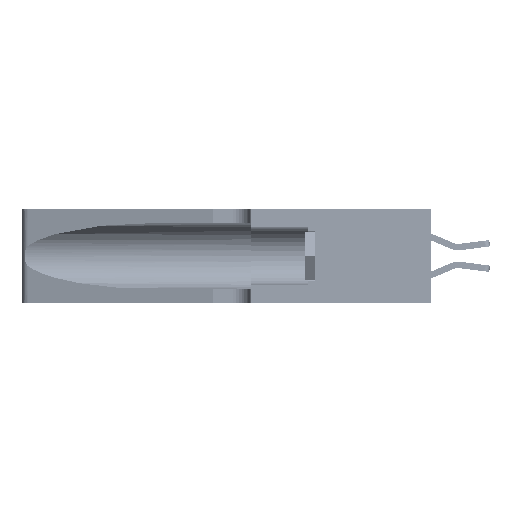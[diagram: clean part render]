
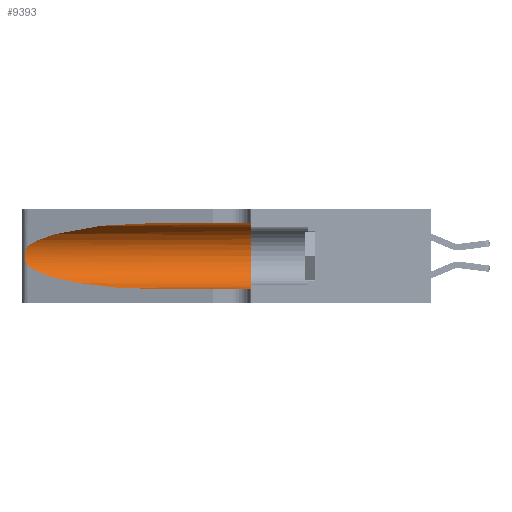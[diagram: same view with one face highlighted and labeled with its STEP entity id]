
A CAD part, left-side view. The second image highlights one B-rep face of the part: STEP entity #9393.
In plain terms, the highlighted cylindrical face has radius 3.308 mm (diameter 6.617 mm), a partial arc.
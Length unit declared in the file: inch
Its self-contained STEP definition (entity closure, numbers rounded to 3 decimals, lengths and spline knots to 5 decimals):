
#1543 = DIRECTION ( 'NONE',  ( 0., 0., 1. ) ) ;
#2768 = AXIS2_PLACEMENT_3D ( 'NONE', #37873, #28418, #1543 ) ;
#3234 = VECTOR ( 'NONE', #26220, 39.37008 ) ;
#3372 = CARTESIAN_POINT ( 'NONE',  ( 0.26017, 1.23833, 0.17102 ) ) ;
#3890 = CARTESIAN_POINT ( 'NONE',  ( 0.25787, 1.23484, 0.2124 ) ) ;
#4260 = VERTEX_POINT ( 'NONE', #5077 ) ;
#5077 = CARTESIAN_POINT ( 'NONE',  ( 0.25487, 1.22718, 0.14631 ) ) ;
#5618 = EDGE_CURVE ( 'NONE', #32539, #18582, #40842, .T. ) ;
#5830 = DIRECTION ( 'NONE',  ( 0., -1., 0. ) ) ;
#6463 = ORIENTED_EDGE ( 'NONE', *, *, #34901, .T. ) ;
#6616 = CARTESIAN_POINT ( 'NONE',  ( 0.18966, 0.96281, 0.31525 ) ) ;
#7053 = ORIENTED_EDGE ( 'NONE', *, *, #42344, .F. ) ;
#7362 = ORIENTED_EDGE ( 'NONE', *, *, #5618, .F. ) ;
#7953 = CARTESIAN_POINT ( 'NONE',  ( 0.25639, 1.23186, 0.15144 ) ) ;
#8888 = CARTESIAN_POINT ( 'NONE',  ( 0.1305, 0.35, 0.31525 ) ) ;
#9348 = CARTESIAN_POINT ( 'NONE',  ( 0.1305, 0.72297, 0.31525 ) ) ;
#9393 = ADVANCED_FACE ( 'NONE', ( #14552 ), #27789, .F. ) ;
#9564 = DIRECTION ( 'NONE',  ( 0., 0., -1. ) ) ;
#11180 = EDGE_CURVE ( 'NONE', #30647, #4260, #34454, .T. ) ;
#14552 = FACE_OUTER_BOUND ( 'NONE', #50273, .T. ) ;
#14632 = CARTESIAN_POINT ( 'NONE',  ( 0.1305, 0.72297, 0.31525 ) ) ;
#15154 = CARTESIAN_POINT ( 'NONE',  ( 0.25487, 1.22718, 0.22369 ) ) ;
#15461 = CARTESIAN_POINT ( 'NONE',  ( 0.25487, 1.22718, 0.22369 ) ) ;
#15671 = DIRECTION ( 'NONE',  ( 0., -1., 0. ) ) ;
#15989 = CARTESIAN_POINT ( 'NONE',  ( 0.26075, 1.23896, 0.19203 ) ) ;
#16619 = CARTESIAN_POINT ( 'NONE',  ( 0.25487, 1.22718, 0.14631 ) ) ;
#17465 = ORIENTED_EDGE ( 'NONE', *, *, #11180, .T. ) ;
#17618 = CARTESIAN_POINT ( 'NONE',  ( 0.1305, 1.61858, 0.05475 ) ) ;
#18582 = VERTEX_POINT ( 'NONE', #36812 ) ;
#19535 = AXIS2_PLACEMENT_3D ( 'NONE', #50505, #5830, #9564 ) ;
#25930 =( BOUNDED_CURVE ( )  B_SPLINE_CURVE ( 3, ( #14632, #6616, #43300, #15154 ),
 .UNSPECIFIED., .F., .F. ) 
 B_SPLINE_CURVE_WITH_KNOTS ( ( 4, 4 ),
 ( 1.5708, 2.84003 ),
 .UNSPECIFIED. ) 
 CURVE ( )  GEOMETRIC_REPRESENTATION_ITEM ( )  RATIONAL_B_SPLINE_CURVE ( ( 1., 0.87, 0.87, 1. ) ) 
 REPRESENTATION_ITEM ( '' )  );
#26193 = VERTEX_POINT ( 'NONE', #9348 ) ;
#26220 = DIRECTION ( 'NONE',  ( 0., -1., 0. ) ) ;
#27789 = CYLINDRICAL_SURFACE ( 'NONE', #19535, 0.13025 ) ;
#27816 = CARTESIAN_POINT ( 'NONE',  ( 0.25856, 1.23593, 0.16098 ) ) ;
#28418 = DIRECTION ( 'NONE',  ( 0., 1., 0. ) ) ;
#29225 = LINE ( 'NONE', #17618, #3234 ) ;
#30647 = VERTEX_POINT ( 'NONE', #37990 ) ;
#30667 = EDGE_CURVE ( 'NONE', #36294, #18582, #29225, .T. ) ;
#31730 = CARTESIAN_POINT ( 'NONE',  ( 0.25789, 1.23486, 0.15765 ) ) ;
#32107 =( BOUNDED_CURVE ( )  B_SPLINE_CURVE ( 3, ( #16619, #44578, #41038, #45284 ),
 .UNSPECIFIED., .F., .F. ) 
 B_SPLINE_CURVE_WITH_KNOTS ( ( 4, 4 ),
 ( 3.44316, 4.71239 ),
 .UNSPECIFIED. ) 
 CURVE ( )  GEOMETRIC_REPRESENTATION_ITEM ( )  RATIONAL_B_SPLINE_CURVE ( ( 1., 0.87, 0.87, 1. ) ) 
 REPRESENTATION_ITEM ( '' )  );
#32539 = VERTEX_POINT ( 'NONE', #8888 ) ;
#34454 = B_SPLINE_CURVE_WITH_KNOTS ( 'NONE', 3,
 ( #15461, #43767, #36178, #3890, #47700, #51940, #15989, #39579, #3372, #27816, #31730, #7953, #35656, #44119 ),
 .UNSPECIFIED., .F., .F.,
 ( 4, 2, 2, 2, 2, 2, 4 ),
 ( 0., 0.00027, 0.00053, 0.00107, 0.0016, 0.00187, 0.00214 ),
 .UNSPECIFIED. ) ;
#34901 = EDGE_CURVE ( 'NONE', #26193, #30647, #25930, .T. ) ;
#35656 = CARTESIAN_POINT ( 'NONE',  ( 0.25555, 1.22993, 0.14849 ) ) ;
#36178 = CARTESIAN_POINT ( 'NONE',  ( 0.25639, 1.23184, 0.21858 ) ) ;
#36294 = VERTEX_POINT ( 'NONE', #40643 ) ;
#36812 = CARTESIAN_POINT ( 'NONE',  ( 0.1305, 0.35, 0.05475 ) ) ;
#37873 = CARTESIAN_POINT ( 'NONE',  ( 0.1305, 0.35, 0.185 ) ) ;
#37990 = CARTESIAN_POINT ( 'NONE',  ( 0.25487, 1.22718, 0.22369 ) ) ;
#38446 = CARTESIAN_POINT ( 'NONE',  ( 0.1305, 1.61858, 0.31525 ) ) ;
#39579 = CARTESIAN_POINT ( 'NONE',  ( 0.26075, 1.23896, 0.178 ) ) ;
#40643 = CARTESIAN_POINT ( 'NONE',  ( 0.1305, 0.72297, 0.05475 ) ) ;
#40842 = CIRCLE ( 'NONE', #2768, 0.13025 ) ;
#41038 = CARTESIAN_POINT ( 'NONE',  ( 0.18966, 0.96281, 0.05475 ) ) ;
#42075 = ORIENTED_EDGE ( 'NONE', *, *, #49332, .T. ) ;
#42344 = EDGE_CURVE ( 'NONE', #26193, #32539, #47414, .T. ) ;
#43300 = CARTESIAN_POINT ( 'NONE',  ( 0.2373, 1.15595, 0.28018 ) ) ;
#43767 = CARTESIAN_POINT ( 'NONE',  ( 0.25555, 1.22994, 0.2215 ) ) ;
#44119 = CARTESIAN_POINT ( 'NONE',  ( 0.25487, 1.22718, 0.14631 ) ) ;
#44578 = CARTESIAN_POINT ( 'NONE',  ( 0.2373, 1.15595, 0.08982 ) ) ;
#45284 = CARTESIAN_POINT ( 'NONE',  ( 0.1305, 0.72297, 0.05475 ) ) ;
#46578 = ORIENTED_EDGE ( 'NONE', *, *, #30667, .T. ) ;
#47414 = LINE ( 'NONE', #38446, #49274 ) ;
#47700 = CARTESIAN_POINT ( 'NONE',  ( 0.25854, 1.2359, 0.20912 ) ) ;
#49274 = VECTOR ( 'NONE', #15671, 39.37008 ) ;
#49332 = EDGE_CURVE ( 'NONE', #4260, #36294, #32107, .T. ) ;
#50273 = EDGE_LOOP ( 'NONE', ( #6463, #17465, #42075, #46578, #7362, #7053 ) ) ;
#50505 = CARTESIAN_POINT ( 'NONE',  ( 0.1305, 1.61858, 0.185 ) ) ;
#51940 = CARTESIAN_POINT ( 'NONE',  ( 0.26018, 1.23835, 0.19895 ) ) ;
